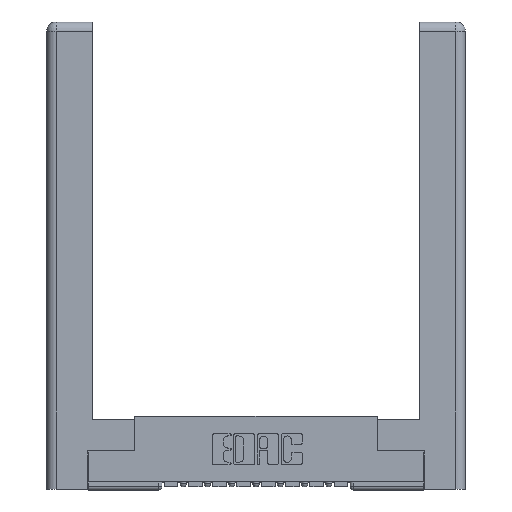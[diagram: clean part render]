
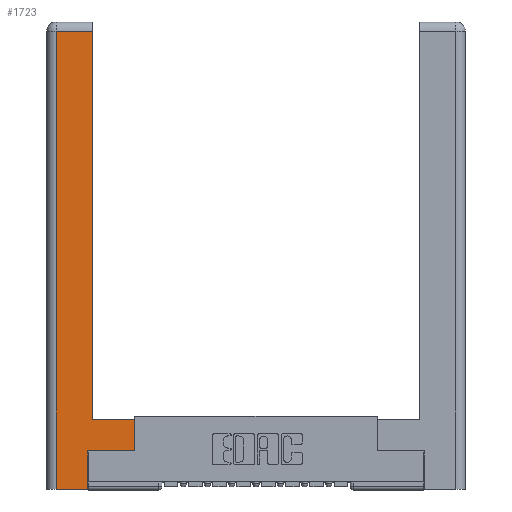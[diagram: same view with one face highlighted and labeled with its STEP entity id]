
A CAD part, top view. The second image highlights one B-rep face of the part: STEP entity #1723.
In plain terms, the highlighted planar face has unit normal (0, 0, 1).
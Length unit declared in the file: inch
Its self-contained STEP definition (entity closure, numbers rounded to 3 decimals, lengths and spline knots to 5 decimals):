
#21 = EDGE_CURVE ( 'NONE', #5425, #3100, #7471, .T. ) ;
#31 = CARTESIAN_POINT ( 'NONE',  ( 0.265, 0., 0. ) ) ;
#344 = ORIENTED_EDGE ( 'NONE', *, *, #2327, .T. ) ;
#467 = EDGE_CURVE ( 'NONE', #5166, #3537, #1601, .T. ) ;
#534 = DIRECTION ( 'NONE',  ( 0., 1., 0. ) ) ;
#604 = PLANE ( 'NONE',  #3312 ) ;
#697 = CARTESIAN_POINT ( 'NONE',  ( 0.295, 0.45, 0. ) ) ;
#1001 = LINE ( 'NONE', #1353, #5069 ) ;
#1176 = LINE ( 'NONE', #6259, #4259 ) ;
#1353 = CARTESIAN_POINT ( 'NONE',  ( 0.0615, 2.94, 0. ) ) ;
#1396 = CARTESIAN_POINT ( 'NONE',  ( 0.0615, 2.94, 0. ) ) ;
#1447 = VECTOR ( 'NONE', #7443, 39.37008 ) ;
#1568 = EDGE_LOOP ( 'NONE', ( #2967, #12666, #3331, #13224, #344, #8221, #6363, #6954 ) ) ;
#1601 = LINE ( 'NONE', #4958, #6377 ) ;
#1723 = ADVANCED_FACE ( 'NONE', ( #6872 ), #604, .F. ) ;
#2219 = CARTESIAN_POINT ( 'NONE',  ( 0.295, 2.94, 0. ) ) ;
#2327 = EDGE_CURVE ( 'NONE', #3100, #11581, #7560, .T. ) ;
#2526 = VERTEX_POINT ( 'NONE', #5966 ) ;
#2878 = CARTESIAN_POINT ( 'NONE',  ( 0., 0., 0. ) ) ;
#2967 = ORIENTED_EDGE ( 'NONE', *, *, #4072, .T. ) ;
#3100 = VERTEX_POINT ( 'NONE', #31 ) ;
#3312 = AXIS2_PLACEMENT_3D ( 'NONE', #2878, #11147, #7670 ) ;
#3331 = ORIENTED_EDGE ( 'NONE', *, *, #10943, .T. ) ;
#3537 = VERTEX_POINT ( 'NONE', #697 ) ;
#4072 = EDGE_CURVE ( 'NONE', #3537, #5362, #1176, .T. ) ;
#4192 = EDGE_CURVE ( 'NONE', #11581, #2526, #10876, .T. ) ;
#4259 = VECTOR ( 'NONE', #534, 39.37008 ) ;
#4464 = VECTOR ( 'NONE', #8445, 39.37008 ) ;
#4515 = CARTESIAN_POINT ( 'NONE',  ( 0.565, 0.245, 0. ) ) ;
#4958 = CARTESIAN_POINT ( 'NONE',  ( 0.295, 0.45, 0. ) ) ;
#5069 = VECTOR ( 'NONE', #13958, 39.37008 ) ;
#5097 = CARTESIAN_POINT ( 'NONE',  ( 0.265, 0., 0. ) ) ;
#5166 = VERTEX_POINT ( 'NONE', #10742 ) ;
#5362 = VERTEX_POINT ( 'NONE', #2219 ) ;
#5425 = VERTEX_POINT ( 'NONE', #12410 ) ;
#5818 = EDGE_CURVE ( 'NONE', #2526, #5166, #7104, .T. ) ;
#5966 = CARTESIAN_POINT ( 'NONE',  ( 0.565, 0.245, 0. ) ) ;
#6259 = CARTESIAN_POINT ( 'NONE',  ( 0.295, 3., 0. ) ) ;
#6363 = ORIENTED_EDGE ( 'NONE', *, *, #5818, .T. ) ;
#6377 = VECTOR ( 'NONE', #8367, 39.37008 ) ;
#6872 = FACE_OUTER_BOUND ( 'NONE', #1568, .T. ) ;
#6954 = ORIENTED_EDGE ( 'NONE', *, *, #467, .T. ) ;
#7104 = LINE ( 'NONE', #9660, #1447 ) ;
#7443 = DIRECTION ( 'NONE',  ( 0., 1., 0. ) ) ;
#7471 = LINE ( 'NONE', #5097, #4464 ) ;
#7560 = LINE ( 'NONE', #13289, #8973 ) ;
#7670 = DIRECTION ( 'NONE',  ( -1., 0., 0. ) ) ;
#8221 = ORIENTED_EDGE ( 'NONE', *, *, #4192, .T. ) ;
#8367 = DIRECTION ( 'NONE',  ( -1., 0., 0. ) ) ;
#8445 = DIRECTION ( 'NONE',  ( 1., 0., 0. ) ) ;
#8690 = LINE ( 'NONE', #13273, #11913 ) ;
#8973 = VECTOR ( 'NONE', #13389, 39.37008 ) ;
#9660 = CARTESIAN_POINT ( 'NONE',  ( 0.565, 0.45, 0. ) ) ;
#10153 = VECTOR ( 'NONE', #14563, 39.37008 ) ;
#10742 = CARTESIAN_POINT ( 'NONE',  ( 0.565, 0.45, 0. ) ) ;
#10876 = LINE ( 'NONE', #4515, #10153 ) ;
#10943 = EDGE_CURVE ( 'NONE', #11168, #5425, #8690, .T. ) ;
#11104 = CARTESIAN_POINT ( 'NONE',  ( 0.265, 0.245, 0. ) ) ;
#11147 = DIRECTION ( 'NONE',  ( 0., 0., -1. ) ) ;
#11168 = VERTEX_POINT ( 'NONE', #1396 ) ;
#11581 = VERTEX_POINT ( 'NONE', #11104 ) ;
#11913 = VECTOR ( 'NONE', #12109, 39.37008 ) ;
#12109 = DIRECTION ( 'NONE',  ( 0., -1., 0. ) ) ;
#12410 = CARTESIAN_POINT ( 'NONE',  ( 0.0615, 0., 0. ) ) ;
#12666 = ORIENTED_EDGE ( 'NONE', *, *, #13934, .T. ) ;
#13224 = ORIENTED_EDGE ( 'NONE', *, *, #21, .T. ) ;
#13273 = CARTESIAN_POINT ( 'NONE',  ( 0.0615, 0., 0. ) ) ;
#13289 = CARTESIAN_POINT ( 'NONE',  ( 0.265, 0.245, 0. ) ) ;
#13389 = DIRECTION ( 'NONE',  ( 0., 1., 0. ) ) ;
#13934 = EDGE_CURVE ( 'NONE', #5362, #11168, #1001, .T. ) ;
#13958 = DIRECTION ( 'NONE',  ( -1., 0., 0. ) ) ;
#14563 = DIRECTION ( 'NONE',  ( 1., 0., 0. ) ) ;
